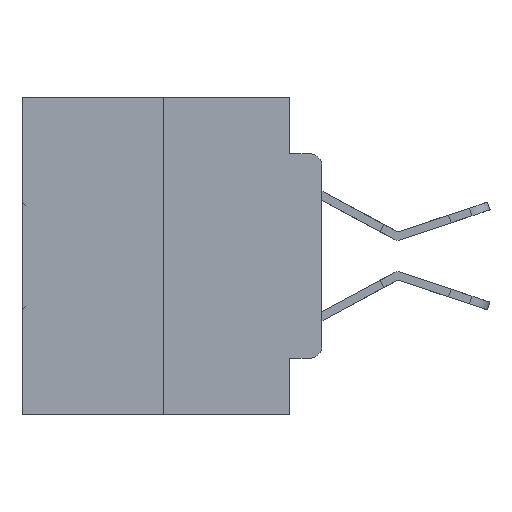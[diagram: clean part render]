
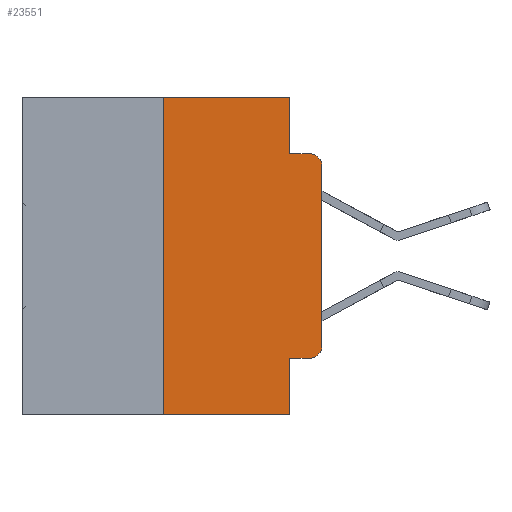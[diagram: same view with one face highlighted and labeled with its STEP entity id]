
A CAD part, left-side view. The second image highlights one B-rep face of the part: STEP entity #23551.
In plain terms, the highlighted planar face has unit normal (-1, 0, 0).
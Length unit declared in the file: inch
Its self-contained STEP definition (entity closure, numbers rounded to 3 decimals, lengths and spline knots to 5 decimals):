
#554 = VERTEX_POINT ( 'NONE', #3531 ) ;
#788 = VECTOR ( 'NONE', #7127, 39.37008 ) ;
#979 = DIRECTION ( 'NONE',  ( 0., -1., 0. ) ) ;
#1201 = CARTESIAN_POINT ( 'NONE',  ( 0., 0., 0. ) ) ;
#1226 = ORIENTED_EDGE ( 'NONE', *, *, #31832, .F. ) ;
#1869 = CARTESIAN_POINT ( 'NONE',  ( 0., 0.02, -0.3915 ) ) ;
#1952 = DIRECTION ( 'NONE',  ( 0., -1., 0. ) ) ;
#2587 = VERTEX_POINT ( 'NONE', #23208 ) ;
#2839 = ORIENTED_EDGE ( 'NONE', *, *, #28618, .T. ) ;
#3069 = EDGE_CURVE ( 'NONE', #21971, #21289, #10181, .T. ) ;
#3510 = VECTOR ( 'NONE', #21901, 39.37008 ) ;
#3531 = CARTESIAN_POINT ( 'NONE',  ( 0., 0.051, 0. ) ) ;
#3634 = PLANE ( 'NONE',  #20752 ) ;
#3892 = VECTOR ( 'NONE', #16365, 39.37008 ) ;
#4031 = ORIENTED_EDGE ( 'NONE', *, *, #8181, .T. ) ;
#4465 = DIRECTION ( 'NONE',  ( 0., 0., -1. ) ) ;
#4816 = EDGE_CURVE ( 'NONE', #554, #5232, #20862, .T. ) ;
#5117 = CARTESIAN_POINT ( 'NONE',  ( 0., 0., -0.3915 ) ) ;
#5232 = VERTEX_POINT ( 'NONE', #21262 ) ;
#5890 = CARTESIAN_POINT ( 'NONE',  ( 0., 0.25, 0. ) ) ;
#6013 = LINE ( 'NONE', #10075, #25061 ) ;
#6183 = DIRECTION ( 'NONE',  ( 0., 0., -1. ) ) ;
#6429 = VECTOR ( 'NONE', #979, 39.37008 ) ;
#6501 = EDGE_CURVE ( 'NONE', #5232, #21404, #29440, .T. ) ;
#6803 = AXIS2_PLACEMENT_3D ( 'NONE', #26703, #11984, #29093 ) ;
#6897 = VERTEX_POINT ( 'NONE', #5117 ) ;
#7062 = CARTESIAN_POINT ( 'NONE',  ( 0., 0.051, 0. ) ) ;
#7102 = CARTESIAN_POINT ( 'NONE',  ( 0., 0.473, -0.5 ) ) ;
#7127 = DIRECTION ( 'NONE',  ( 0., 0., -1. ) ) ;
#7463 = EDGE_LOOP ( 'NONE', ( #13037, #4031, #17444, #12386, #18972, #19745, #26966, #1226, #7991, #2839 ) ) ;
#7991 = ORIENTED_EDGE ( 'NONE', *, *, #30222, .T. ) ;
#8022 = CARTESIAN_POINT ( 'NONE',  ( 0., 0.051, -0.4115 ) ) ;
#8181 = EDGE_CURVE ( 'NONE', #22037, #21404, #25966, .T. ) ;
#8796 = LINE ( 'NONE', #13673, #6429 ) ;
#8874 = CARTESIAN_POINT ( 'NONE',  ( 0., 0.02, -0.0885 ) ) ;
#9907 = EDGE_CURVE ( 'NONE', #6897, #22037, #23212, .T. ) ;
#10075 = CARTESIAN_POINT ( 'NONE',  ( 0., 0.473, 0. ) ) ;
#10132 = LINE ( 'NONE', #7102, #29674 ) ;
#10181 = LINE ( 'NONE', #20618, #23355 ) ;
#10295 = LINE ( 'NONE', #16956, #3510 ) ;
#11984 = DIRECTION ( 'NONE',  ( -1., 0., 0. ) ) ;
#12386 = ORIENTED_EDGE ( 'NONE', *, *, #4816, .F. ) ;
#13037 = ORIENTED_EDGE ( 'NONE', *, *, #9907, .T. ) ;
#13673 = CARTESIAN_POINT ( 'NONE',  ( 0., 0.051, -0.4115 ) ) ;
#13946 = CARTESIAN_POINT ( 'NONE',  ( 0., 0.25, -0.5 ) ) ;
#16348 = CIRCLE ( 'NONE', #29349, 0.02 ) ;
#16365 = DIRECTION ( 'NONE',  ( 0., -1., 0. ) ) ;
#16591 = VERTEX_POINT ( 'NONE', #8022 ) ;
#16956 = CARTESIAN_POINT ( 'NONE',  ( 0., 0.051, 0. ) ) ;
#17444 = ORIENTED_EDGE ( 'NONE', *, *, #6501, .F. ) ;
#17838 = CARTESIAN_POINT ( 'NONE',  ( 0., 0.051, -0.5 ) ) ;
#18389 = VERTEX_POINT ( 'NONE', #17838 ) ;
#18972 = ORIENTED_EDGE ( 'NONE', *, *, #27856, .F. ) ;
#19474 = DIRECTION ( 'NONE',  ( -1., 0., 0. ) ) ;
#19745 = ORIENTED_EDGE ( 'NONE', *, *, #3069, .F. ) ;
#20618 = CARTESIAN_POINT ( 'NONE',  ( 0., 0.25, 0. ) ) ;
#20752 = AXIS2_PLACEMENT_3D ( 'NONE', #23508, #21156, #6183 ) ;
#20862 = LINE ( 'NONE', #7062, #788 ) ;
#21156 = DIRECTION ( 'NONE',  ( 1., 0., 0. ) ) ;
#21262 = CARTESIAN_POINT ( 'NONE',  ( 0., 0.051, -0.0885 ) ) ;
#21289 = VERTEX_POINT ( 'NONE', #5890 ) ;
#21404 = VERTEX_POINT ( 'NONE', #8874 ) ;
#21901 = DIRECTION ( 'NONE',  ( 0., 0., -1. ) ) ;
#21971 = VERTEX_POINT ( 'NONE', #13946 ) ;
#22037 = VERTEX_POINT ( 'NONE', #23935 ) ;
#22906 = DIRECTION ( 'NONE',  ( 0., 0., 1. ) ) ;
#23208 = CARTESIAN_POINT ( 'NONE',  ( 0., 0.02, -0.4115 ) ) ;
#23212 = LINE ( 'NONE', #1201, #28828 ) ;
#23355 = VECTOR ( 'NONE', #22906, 39.37008 ) ;
#23508 = CARTESIAN_POINT ( 'NONE',  ( 0., 0.473, 0. ) ) ;
#23551 = ADVANCED_FACE ( 'NONE', ( #31342 ), #3634, .F. ) ;
#23935 = CARTESIAN_POINT ( 'NONE',  ( 0., 0., -0.1085 ) ) ;
#25061 = VECTOR ( 'NONE', #27285, 39.37008 ) ;
#25838 = EDGE_CURVE ( 'NONE', #21971, #18389, #10132, .T. ) ;
#25966 = CIRCLE ( 'NONE', #6803, 0.02 ) ;
#26175 = CARTESIAN_POINT ( 'NONE',  ( 0., 0.051, -0.0885 ) ) ;
#26703 = CARTESIAN_POINT ( 'NONE',  ( 0., 0.02, -0.1085 ) ) ;
#26966 = ORIENTED_EDGE ( 'NONE', *, *, #25838, .T. ) ;
#27285 = DIRECTION ( 'NONE',  ( 0., -1., 0. ) ) ;
#27856 = EDGE_CURVE ( 'NONE', #21289, #554, #6013, .T. ) ;
#28618 = EDGE_CURVE ( 'NONE', #2587, #6897, #16348, .T. ) ;
#28828 = VECTOR ( 'NONE', #30889, 39.37008 ) ;
#29093 = DIRECTION ( 'NONE',  ( 0., 0., -1. ) ) ;
#29349 = AXIS2_PLACEMENT_3D ( 'NONE', #1869, #19474, #4465 ) ;
#29440 = LINE ( 'NONE', #26175, #3892 ) ;
#29674 = VECTOR ( 'NONE', #1952, 39.37008 ) ;
#30222 = EDGE_CURVE ( 'NONE', #16591, #2587, #8796, .T. ) ;
#30889 = DIRECTION ( 'NONE',  ( 0., 0., 1. ) ) ;
#31342 = FACE_OUTER_BOUND ( 'NONE', #7463, .T. ) ;
#31832 = EDGE_CURVE ( 'NONE', #16591, #18389, #10295, .T. ) ;
